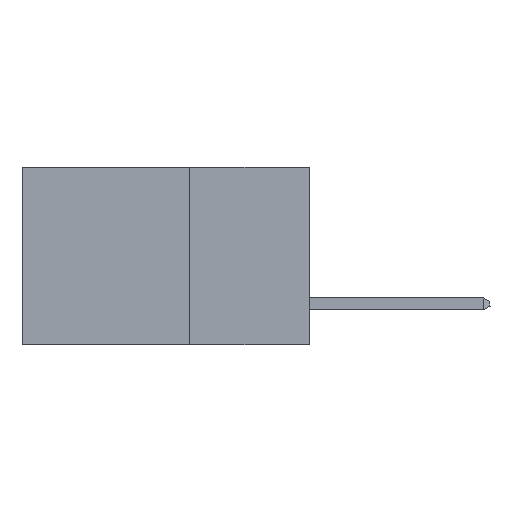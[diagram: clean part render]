
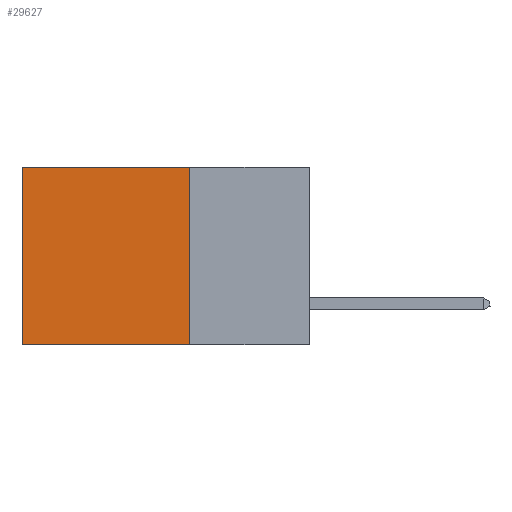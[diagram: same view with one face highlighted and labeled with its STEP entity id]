
A CAD part, left-side view. The second image highlights one B-rep face of the part: STEP entity #29627.
In plain terms, the highlighted planar face has unit normal (-1, 0, 0).
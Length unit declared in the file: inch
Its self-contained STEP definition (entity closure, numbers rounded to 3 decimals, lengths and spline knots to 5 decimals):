
#887 = VERTEX_POINT ( 'NONE', #4230 ) ;
#3414 = FACE_OUTER_BOUND ( 'NONE', #8753, .T. ) ;
#3680 = EDGE_CURVE ( 'NONE', #5528, #8388, #37960, .T. ) ;
#4230 = CARTESIAN_POINT ( 'NONE',  ( 0.2875, 0.25, 0. ) ) ;
#5016 = DIRECTION ( 'NONE',  ( 0., 0., -1. ) ) ;
#5211 = CARTESIAN_POINT ( 'NONE',  ( 0.2875, 0.25, 0. ) ) ;
#5528 = VERTEX_POINT ( 'NONE', #27082 ) ;
#6075 = DIRECTION ( 'NONE',  ( 1., 0., 0. ) ) ;
#7574 = VECTOR ( 'NONE', #23009, 39.37008 ) ;
#8138 = ORIENTED_EDGE ( 'NONE', *, *, #3680, .T. ) ;
#8388 = VERTEX_POINT ( 'NONE', #43871 ) ;
#8753 = EDGE_LOOP ( 'NONE', ( #8138, #15712, #23068, #35216 ) ) ;
#10861 = DIRECTION ( 'NONE',  ( 0., 0., -1. ) ) ;
#11944 = LINE ( 'NONE', #5211, #7574 ) ;
#12761 = VECTOR ( 'NONE', #5016, 39.37008 ) ;
#14022 = DIRECTION ( 'NONE',  ( 0., 1., 0. ) ) ;
#14229 = CARTESIAN_POINT ( 'NONE',  ( 0.2875, 0.25, 0. ) ) ;
#15171 = DIRECTION ( 'NONE',  ( 0., 1., 0. ) ) ;
#15712 = ORIENTED_EDGE ( 'NONE', *, *, #39308, .F. ) ;
#17392 = LINE ( 'NONE', #39525, #46730 ) ;
#17421 = VERTEX_POINT ( 'NONE', #38779 ) ;
#18777 = LINE ( 'NONE', #40902, #36998 ) ;
#23009 = DIRECTION ( 'NONE',  ( 0., 0., -1. ) ) ;
#23068 = ORIENTED_EDGE ( 'NONE', *, *, #37504, .F. ) ;
#25464 = AXIS2_PLACEMENT_3D ( 'NONE', #14229, #6075, #10861 ) ;
#27082 = CARTESIAN_POINT ( 'NONE',  ( 0.2875, 0.6, 0. ) ) ;
#29627 = ADVANCED_FACE ( 'NONE', ( #3414 ), #32525, .F. ) ;
#29722 = EDGE_CURVE ( 'NONE', #887, #5528, #18777, .T. ) ;
#32525 = PLANE ( 'NONE',  #25464 ) ;
#34337 = CARTESIAN_POINT ( 'NONE',  ( 0.2875, 0.6, 0. ) ) ;
#35216 = ORIENTED_EDGE ( 'NONE', *, *, #29722, .T. ) ;
#36998 = VECTOR ( 'NONE', #15171, 39.37008 ) ;
#37504 = EDGE_CURVE ( 'NONE', #887, #17421, #11944, .T. ) ;
#37960 = LINE ( 'NONE', #34337, #12761 ) ;
#38779 = CARTESIAN_POINT ( 'NONE',  ( 0.2875, 0.25, -0.37 ) ) ;
#39308 = EDGE_CURVE ( 'NONE', #17421, #8388, #17392, .T. ) ;
#39525 = CARTESIAN_POINT ( 'NONE',  ( 0.2875, 0.25, -0.37 ) ) ;
#40902 = CARTESIAN_POINT ( 'NONE',  ( 0.2875, 0.25, 0. ) ) ;
#43871 = CARTESIAN_POINT ( 'NONE',  ( 0.2875, 0.6, -0.37 ) ) ;
#46730 = VECTOR ( 'NONE', #14022, 39.37008 ) ;
